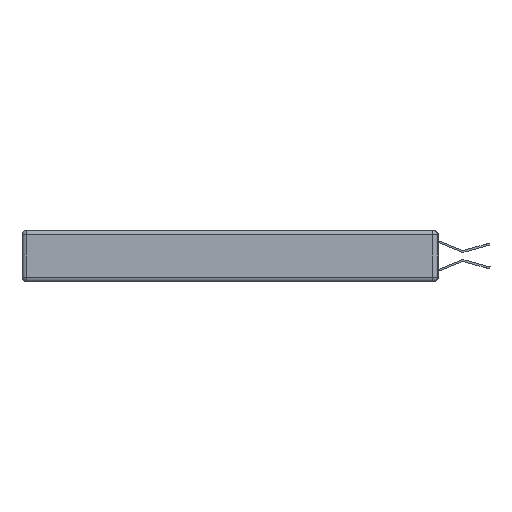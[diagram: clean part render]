
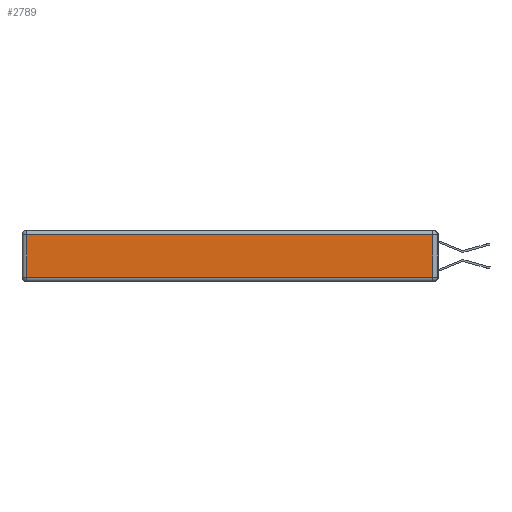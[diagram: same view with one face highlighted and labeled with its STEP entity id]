
A CAD part, left-side view. The second image highlights one B-rep face of the part: STEP entity #2789.
In plain terms, the highlighted planar face has unit normal (-1, 0, 0).
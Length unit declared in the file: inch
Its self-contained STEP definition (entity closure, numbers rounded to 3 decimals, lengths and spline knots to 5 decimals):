
#24 = DIRECTION ( 'NONE',  ( 0., -1., 0. ) ) ;
#381 = CARTESIAN_POINT ( 'NONE',  ( 0., 2.75, -0.03 ) ) ;
#776 = VERTEX_POINT ( 'NONE', #3313 ) ;
#1547 = VECTOR ( 'NONE', #13499, 39.37008 ) ;
#2093 = ORIENTED_EDGE ( 'NONE', *, *, #12273, .T. ) ;
#2789 = ADVANCED_FACE ( 'NONE', ( #8214 ), #15413, .T. ) ;
#3119 = LINE ( 'NONE', #8677, #7864 ) ;
#3198 = VECTOR ( 'NONE', #13437, 39.37008 ) ;
#3313 = CARTESIAN_POINT ( 'NONE',  ( 0., 2.72, -0.03 ) ) ;
#3331 = CARTESIAN_POINT ( 'NONE',  ( 0., 0.03, -0.343 ) ) ;
#3966 = DIRECTION ( 'NONE',  ( -1., 0., 0. ) ) ;
#4024 = DIRECTION ( 'NONE',  ( 0., 0., 1. ) ) ;
#4332 = VERTEX_POINT ( 'NONE', #10245 ) ;
#5110 = EDGE_CURVE ( 'NONE', #7529, #4332, #3119, .T. ) ;
#5269 = EDGE_LOOP ( 'NONE', ( #10067, #8228, #9710, #2093 ) ) ;
#5313 = LINE ( 'NONE', #381, #1547 ) ;
#7039 = LINE ( 'NONE', #3331, #3198 ) ;
#7529 = VERTEX_POINT ( 'NONE', #18029 ) ;
#7864 = VECTOR ( 'NONE', #24, 39.37008 ) ;
#8214 = FACE_OUTER_BOUND ( 'NONE', #5269, .T. ) ;
#8228 = ORIENTED_EDGE ( 'NONE', *, *, #11462, .T. ) ;
#8677 = CARTESIAN_POINT ( 'NONE',  ( 0., 0., -0.313 ) ) ;
#9710 = ORIENTED_EDGE ( 'NONE', *, *, #13284, .T. ) ;
#9971 = AXIS2_PLACEMENT_3D ( 'NONE', #14208, #3966, #4024 ) ;
#10067 = ORIENTED_EDGE ( 'NONE', *, *, #5110, .T. ) ;
#10245 = CARTESIAN_POINT ( 'NONE',  ( 0., 0.03, -0.313 ) ) ;
#10630 = LINE ( 'NONE', #14240, #18358 ) ;
#11410 = DIRECTION ( 'NONE',  ( 0., 0., -1. ) ) ;
#11462 = EDGE_CURVE ( 'NONE', #4332, #12908, #7039, .T. ) ;
#12273 = EDGE_CURVE ( 'NONE', #776, #7529, #10630, .T. ) ;
#12908 = VERTEX_POINT ( 'NONE', #14151 ) ;
#13284 = EDGE_CURVE ( 'NONE', #12908, #776, #5313, .T. ) ;
#13437 = DIRECTION ( 'NONE',  ( 0., 0., 1. ) ) ;
#13499 = DIRECTION ( 'NONE',  ( 0., 1., 0. ) ) ;
#14151 = CARTESIAN_POINT ( 'NONE',  ( 0., 0.03, -0.03 ) ) ;
#14208 = CARTESIAN_POINT ( 'NONE',  ( 0., 0., -0.343 ) ) ;
#14240 = CARTESIAN_POINT ( 'NONE',  ( 0., 2.72, -0.343 ) ) ;
#15413 = PLANE ( 'NONE',  #9971 ) ;
#18029 = CARTESIAN_POINT ( 'NONE',  ( 0., 2.72, -0.313 ) ) ;
#18358 = VECTOR ( 'NONE', #11410, 39.37008 ) ;
